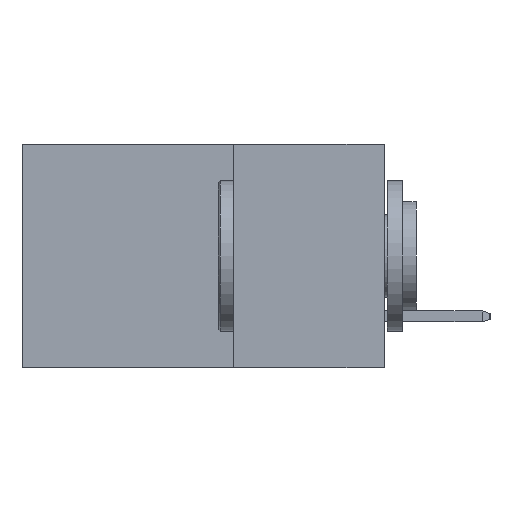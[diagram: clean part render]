
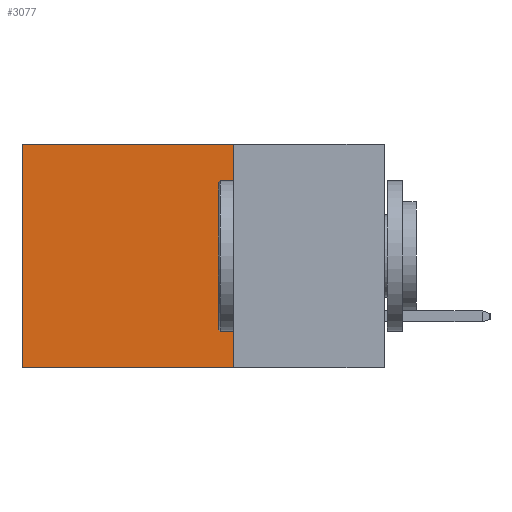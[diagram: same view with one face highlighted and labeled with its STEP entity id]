
A CAD part, left-side view. The second image highlights one B-rep face of the part: STEP entity #3077.
In plain terms, the highlighted planar face has unit normal (-1, 0, 0).
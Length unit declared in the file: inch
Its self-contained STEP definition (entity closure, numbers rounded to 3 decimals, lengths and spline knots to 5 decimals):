
#1885 = DIRECTION ( 'NONE',  ( 0., 0., -1. ) ) ;
#2335 = VERTEX_POINT ( 'NONE', #26236 ) ;
#3077 = ADVANCED_FACE ( 'NONE', ( #26598 ), #24073, .F. ) ;
#3803 = VECTOR ( 'NONE', #12262, 39.37008 ) ;
#3865 = DIRECTION ( 'NONE',  ( 0., 1., 0. ) ) ;
#4583 = LINE ( 'NONE', #24600, #3803 ) ;
#4632 = CARTESIAN_POINT ( 'NONE',  ( 0.298, 0.25, 0. ) ) ;
#4640 = EDGE_CURVE ( 'NONE', #2335, #24899, #11449, .T. ) ;
#6247 = EDGE_CURVE ( 'NONE', #18410, #24899, #16654, .T. ) ;
#6760 = CARTESIAN_POINT ( 'NONE',  ( 0.298, 0.25, 0. ) ) ;
#9610 = CARTESIAN_POINT ( 'NONE',  ( 0.298, 0.25, -0.37 ) ) ;
#10870 = ORIENTED_EDGE ( 'NONE', *, *, #28517, .T. ) ;
#10915 = AXIS2_PLACEMENT_3D ( 'NONE', #6760, #16714, #1885 ) ;
#11449 = LINE ( 'NONE', #29415, #23854 ) ;
#11842 = LINE ( 'NONE', #18673, #19224 ) ;
#12020 = ORIENTED_EDGE ( 'NONE', *, *, #19077, .F. ) ;
#12195 = DIRECTION ( 'NONE',  ( 0., 0., -1. ) ) ;
#12262 = DIRECTION ( 'NONE',  ( 0., 0., -1. ) ) ;
#13060 = CARTESIAN_POINT ( 'NONE',  ( 0.298, 0.25, -0.37 ) ) ;
#13762 = EDGE_LOOP ( 'NONE', ( #25325, #27403, #12020, #10870 ) ) ;
#15557 = DIRECTION ( 'NONE',  ( 0., 1., 0. ) ) ;
#16654 = LINE ( 'NONE', #13060, #28962 ) ;
#16714 = DIRECTION ( 'NONE',  ( 1., 0., 0. ) ) ;
#18410 = VERTEX_POINT ( 'NONE', #9610 ) ;
#18673 = CARTESIAN_POINT ( 'NONE',  ( 0.298, 0.25, 0. ) ) ;
#19077 = EDGE_CURVE ( 'NONE', #20463, #18410, #4583, .T. ) ;
#19224 = VECTOR ( 'NONE', #3865, 39.37008 ) ;
#20463 = VERTEX_POINT ( 'NONE', #4632 ) ;
#23854 = VECTOR ( 'NONE', #12195, 39.37008 ) ;
#24073 = PLANE ( 'NONE',  #10915 ) ;
#24600 = CARTESIAN_POINT ( 'NONE',  ( 0.298, 0.25, 0. ) ) ;
#24899 = VERTEX_POINT ( 'NONE', #31916 ) ;
#25325 = ORIENTED_EDGE ( 'NONE', *, *, #4640, .T. ) ;
#26236 = CARTESIAN_POINT ( 'NONE',  ( 0.298, 0.6, 0. ) ) ;
#26598 = FACE_OUTER_BOUND ( 'NONE', #13762, .T. ) ;
#27403 = ORIENTED_EDGE ( 'NONE', *, *, #6247, .F. ) ;
#28517 = EDGE_CURVE ( 'NONE', #20463, #2335, #11842, .T. ) ;
#28962 = VECTOR ( 'NONE', #15557, 39.37008 ) ;
#29415 = CARTESIAN_POINT ( 'NONE',  ( 0.298, 0.6, 0. ) ) ;
#31916 = CARTESIAN_POINT ( 'NONE',  ( 0.298, 0.6, -0.37 ) ) ;
